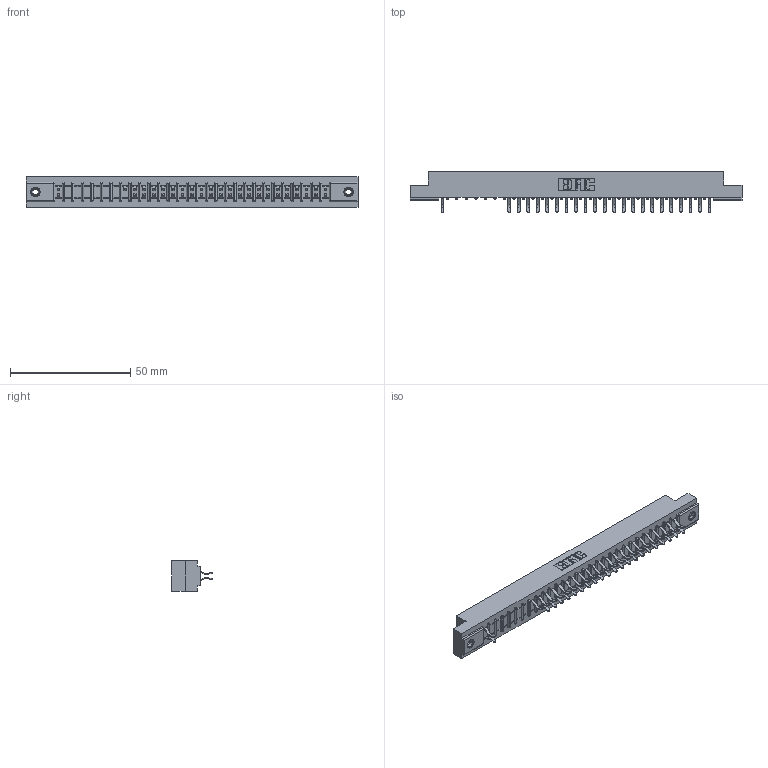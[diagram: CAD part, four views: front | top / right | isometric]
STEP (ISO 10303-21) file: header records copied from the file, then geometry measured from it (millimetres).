
FILE_DESCRIPTION (( 'STEP AP203' ), '1' );
FILE_NAME ('307-058-556-208.STEP', '2018-08-06T07:50:32', ( '' ), ( '' ), 'SwSTEP 2.0', 'SolidWorks 2016', '' );
FILE_SCHEMA (( 'CONFIG_CONTROL_DESIGN' ));
Length unit declared in the file: inch
Products named in the file (4): 307-058-556-208; 307 Part_.156 Dia Mounting Holes; 307-290-001_556; 345-250-001_345-250-003-102
Assembly tree (48 placements, depth 2):
  307-058-556-208
    307 Part_.156 Dia Mounting Holes
    307-290-001_556  x45
    345-250-001_345-250-003-102  x2
Bounding box: 137.92 x 16.97 x 12.7 mm (x, y, z)
Volume: 14391.3 mm3; surface area: 16142.9 mm2
Topology: 48 solids, 48 shells, 2588 faces, 7265 edges, 4694 vertices
Faces by surface type: plane 1665, cylinder 847, sphere 60, cone 12, torus 4
Entity records: 28265 total; most frequent: CARTESIAN_POINT 4667, ORIENTED_EDGE 4630, DIRECTION 4573, EDGE_CURVE 2315, VECTOR 1769, LINE 1769, VERTEX_POINT 1496, AXIS2_PLACEMENT_3D 1402
